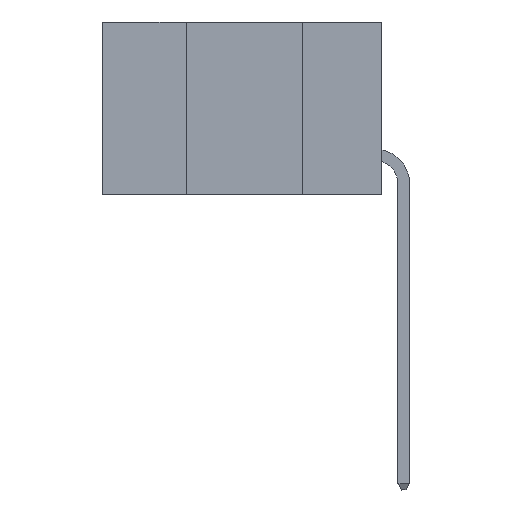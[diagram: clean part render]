
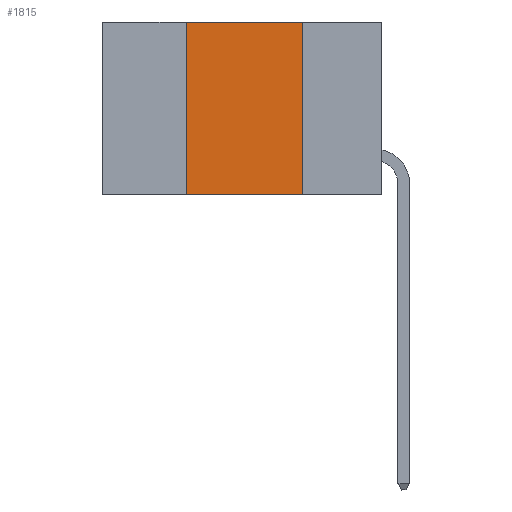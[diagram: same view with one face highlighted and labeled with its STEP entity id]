
A CAD part, left-side view. The second image highlights one B-rep face of the part: STEP entity #1815.
In plain terms, the highlighted planar face has unit normal (-1, 0, 0).
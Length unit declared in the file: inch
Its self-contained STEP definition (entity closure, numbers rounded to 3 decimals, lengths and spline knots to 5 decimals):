
#264 = LINE ( 'NONE', #8782, #18713 ) ;
#361 = DIRECTION ( 'NONE',  ( 1., 0., 0. ) ) ;
#1455 = ORIENTED_EDGE ( 'NONE', *, *, #14856, .F. ) ;
#1815 = ADVANCED_FACE ( 'NONE', ( #26452 ), #14137, .F. ) ;
#2736 = DIRECTION ( 'NONE',  ( 0., 0., -1. ) ) ;
#3269 = EDGE_CURVE ( 'NONE', #14150, #11033, #24227, .T. ) ;
#4264 = CARTESIAN_POINT ( 'NONE',  ( 0., 0.42, 0. ) ) ;
#4586 = VECTOR ( 'NONE', #5289, 39.37008 ) ;
#5289 = DIRECTION ( 'NONE',  ( 0., 0., -1. ) ) ;
#5466 = DIRECTION ( 'NONE',  ( 0., 0., 1. ) ) ;
#6267 = CARTESIAN_POINT ( 'NONE',  ( 0., 0.17, -0.37 ) ) ;
#6352 = CARTESIAN_POINT ( 'NONE',  ( 0., 0.42, -0.37 ) ) ;
#8305 = VERTEX_POINT ( 'NONE', #21952 ) ;
#8782 = CARTESIAN_POINT ( 'NONE',  ( 0., 0.6, 0. ) ) ;
#11033 = VERTEX_POINT ( 'NONE', #6267 ) ;
#12226 = CARTESIAN_POINT ( 'NONE',  ( 0., 0.17, 0. ) ) ;
#12845 = CARTESIAN_POINT ( 'NONE',  ( 0., 0.42, 0. ) ) ;
#13347 = DIRECTION ( 'NONE',  ( 0., -1., 0. ) ) ;
#13860 = EDGE_CURVE ( 'NONE', #8305, #11033, #15933, .T. ) ;
#14026 = VECTOR ( 'NONE', #26527, 39.37008 ) ;
#14137 = PLANE ( 'NONE',  #19105 ) ;
#14150 = VERTEX_POINT ( 'NONE', #6352 ) ;
#14606 = CARTESIAN_POINT ( 'NONE',  ( 0., 0.6, -0.37 ) ) ;
#14856 = EDGE_CURVE ( 'NONE', #22686, #8305, #264, .T. ) ;
#15933 = LINE ( 'NONE', #12226, #4586 ) ;
#16508 = CARTESIAN_POINT ( 'NONE',  ( 0., 0.6, 0. ) ) ;
#18713 = VECTOR ( 'NONE', #13347, 39.37008 ) ;
#19105 = AXIS2_PLACEMENT_3D ( 'NONE', #16508, #361, #2736 ) ;
#20830 = LINE ( 'NONE', #4264, #26809 ) ;
#21590 = ORIENTED_EDGE ( 'NONE', *, *, #22112, .F. ) ;
#21952 = CARTESIAN_POINT ( 'NONE',  ( 0., 0.17, 0. ) ) ;
#22112 = EDGE_CURVE ( 'NONE', #14150, #22686, #20830, .T. ) ;
#22686 = VERTEX_POINT ( 'NONE', #12845 ) ;
#23814 = ORIENTED_EDGE ( 'NONE', *, *, #13860, .F. ) ;
#24227 = LINE ( 'NONE', #14606, #14026 ) ;
#24944 = EDGE_LOOP ( 'NONE', ( #23814, #1455, #21590, #28908 ) ) ;
#26452 = FACE_OUTER_BOUND ( 'NONE', #24944, .T. ) ;
#26527 = DIRECTION ( 'NONE',  ( 0., -1., 0. ) ) ;
#26809 = VECTOR ( 'NONE', #5466, 39.37008 ) ;
#28908 = ORIENTED_EDGE ( 'NONE', *, *, #3269, .T. ) ;
